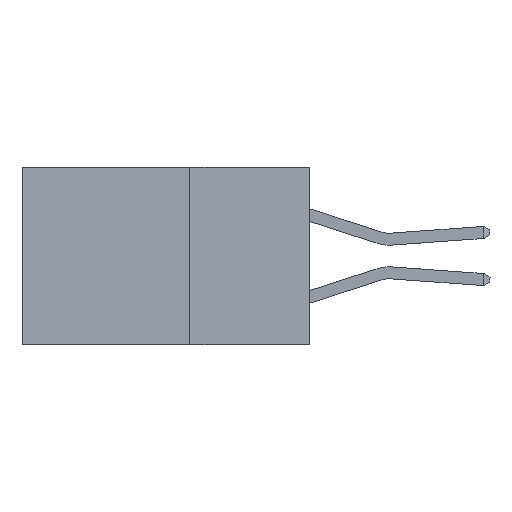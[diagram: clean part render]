
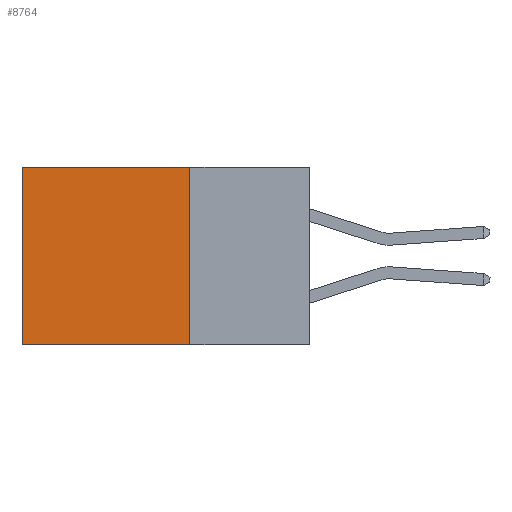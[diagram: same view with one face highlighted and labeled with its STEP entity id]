
A CAD part, left-side view. The second image highlights one B-rep face of the part: STEP entity #8764.
In plain terms, the highlighted planar face has unit normal (-1, 0, 0).
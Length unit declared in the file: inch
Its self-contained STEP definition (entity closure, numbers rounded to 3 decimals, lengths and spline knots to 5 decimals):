
#1387 = ORIENTED_EDGE ( 'NONE', *, *, #7731, .T. ) ;
#1551 = DIRECTION ( 'NONE',  ( 1., 0., 0. ) ) ;
#2089 = AXIS2_PLACEMENT_3D ( 'NONE', #24992, #1551, #15292 ) ;
#3052 = CARTESIAN_POINT ( 'NONE',  ( 0.2615, 0.25, 0. ) ) ;
#3343 = CARTESIAN_POINT ( 'NONE',  ( 0.2615, 0.6, 0. ) ) ;
#3669 = DIRECTION ( 'NONE',  ( 0., 1., 0. ) ) ;
#3752 = CARTESIAN_POINT ( 'NONE',  ( 0.2615, 0.25, -0.37 ) ) ;
#4508 = EDGE_CURVE ( 'NONE', #18015, #8395, #8000, .T. ) ;
#6910 = LINE ( 'NONE', #13163, #21898 ) ;
#6916 = LINE ( 'NONE', #17498, #16724 ) ;
#7731 = EDGE_CURVE ( 'NONE', #11836, #20518, #6916, .T. ) ;
#8000 = LINE ( 'NONE', #3752, #18440 ) ;
#8395 = VERTEX_POINT ( 'NONE', #18077 ) ;
#8764 = ADVANCED_FACE ( 'NONE', ( #25197 ), #11342, .F. ) ;
#10217 = LINE ( 'NONE', #14696, #15440 ) ;
#10745 = ORIENTED_EDGE ( 'NONE', *, *, #4508, .F. ) ;
#11072 = CARTESIAN_POINT ( 'NONE',  ( 0.2615, 0.25, -0.37 ) ) ;
#11342 = PLANE ( 'NONE',  #2089 ) ;
#11836 = VERTEX_POINT ( 'NONE', #3052 ) ;
#12578 = ORIENTED_EDGE ( 'NONE', *, *, #14252, .T. ) ;
#13163 = CARTESIAN_POINT ( 'NONE',  ( 0.2615, 0.6, -0.37 ) ) ;
#14252 = EDGE_CURVE ( 'NONE', #20518, #8395, #6910, .T. ) ;
#14518 = EDGE_LOOP ( 'NONE', ( #12578, #10745, #22364, #1387 ) ) ;
#14696 = CARTESIAN_POINT ( 'NONE',  ( 0.2615, 0.25, -0.37 ) ) ;
#15124 = DIRECTION ( 'NONE',  ( 0., 0., -1. ) ) ;
#15292 = DIRECTION ( 'NONE',  ( 0., 0., -1. ) ) ;
#15440 = VECTOR ( 'NONE', #24393, 39.37008 ) ;
#16724 = VECTOR ( 'NONE', #19461, 39.37008 ) ;
#17498 = CARTESIAN_POINT ( 'NONE',  ( 0.2615, 0.25, 0. ) ) ;
#18015 = VERTEX_POINT ( 'NONE', #11072 ) ;
#18077 = CARTESIAN_POINT ( 'NONE',  ( 0.2615, 0.6, -0.37 ) ) ;
#18440 = VECTOR ( 'NONE', #3669, 39.37008 ) ;
#19461 = DIRECTION ( 'NONE',  ( 0., 1., 0. ) ) ;
#20518 = VERTEX_POINT ( 'NONE', #3343 ) ;
#21898 = VECTOR ( 'NONE', #15124, 39.37008 ) ;
#22364 = ORIENTED_EDGE ( 'NONE', *, *, #23624, .F. ) ;
#23624 = EDGE_CURVE ( 'NONE', #11836, #18015, #10217, .T. ) ;
#24393 = DIRECTION ( 'NONE',  ( 0., 0., -1. ) ) ;
#24992 = CARTESIAN_POINT ( 'NONE',  ( 0.2615, 0.25, -0.37 ) ) ;
#25197 = FACE_OUTER_BOUND ( 'NONE', #14518, .T. ) ;
